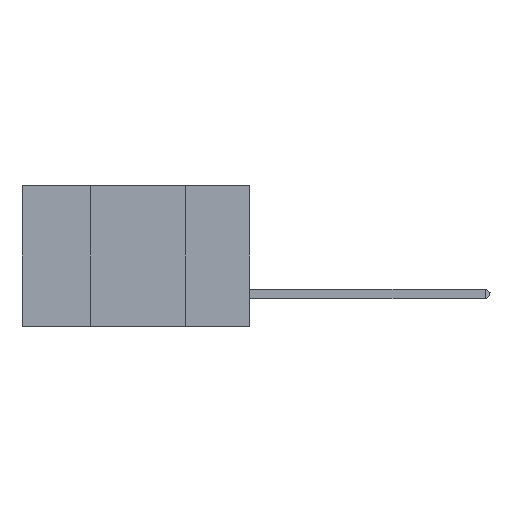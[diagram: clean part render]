
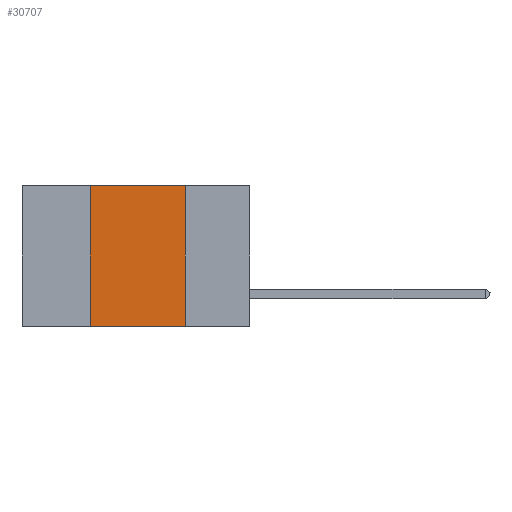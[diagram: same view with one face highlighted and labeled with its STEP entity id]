
A CAD part, left-side view. The second image highlights one B-rep face of the part: STEP entity #30707.
In plain terms, the highlighted planar face has unit normal (-1, 0, 0).
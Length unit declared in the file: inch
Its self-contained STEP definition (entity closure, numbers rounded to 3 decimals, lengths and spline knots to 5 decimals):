
#6168 = CARTESIAN_POINT ( 'NONE',  ( 0., 0.6, 0. ) ) ;
#6677 = ORIENTED_EDGE ( 'NONE', *, *, #27376, .F. ) ;
#6798 = VERTEX_POINT ( 'NONE', #9620 ) ;
#7410 = ORIENTED_EDGE ( 'NONE', *, *, #22093, .T. ) ;
#7739 = CARTESIAN_POINT ( 'NONE',  ( 0., 0.6, -0.37 ) ) ;
#8083 = CARTESIAN_POINT ( 'NONE',  ( 0., 0.17, 0. ) ) ;
#8646 = VERTEX_POINT ( 'NONE', #12746 ) ;
#9620 = CARTESIAN_POINT ( 'NONE',  ( 0., 0.42, 0. ) ) ;
#10170 = EDGE_CURVE ( 'NONE', #6798, #12693, #30324, .T. ) ;
#10676 = LINE ( 'NONE', #17947, #24309 ) ;
#11030 = VECTOR ( 'NONE', #15899, 39.37008 ) ;
#11172 = PLANE ( 'NONE',  #33672 ) ;
#12693 = VERTEX_POINT ( 'NONE', #8083 ) ;
#12746 = CARTESIAN_POINT ( 'NONE',  ( 0., 0.17, -0.37 ) ) ;
#14171 = DIRECTION ( 'NONE',  ( 0., 0., -1. ) ) ;
#14603 = VECTOR ( 'NONE', #25140, 39.37008 ) ;
#14664 = CARTESIAN_POINT ( 'NONE',  ( 0., 0.6, 0. ) ) ;
#15554 = ORIENTED_EDGE ( 'NONE', *, *, #22669, .F. ) ;
#15651 = EDGE_LOOP ( 'NONE', ( #15554, #31844, #6677, #7410 ) ) ;
#15899 = DIRECTION ( 'NONE',  ( 0., -1., 0. ) ) ;
#17947 = CARTESIAN_POINT ( 'NONE',  ( 0., 0.42, 0. ) ) ;
#18639 = FACE_OUTER_BOUND ( 'NONE', #15651, .T. ) ;
#20091 = LINE ( 'NONE', #23366, #29177 ) ;
#22093 = EDGE_CURVE ( 'NONE', #28716, #8646, #30490, .T. ) ;
#22669 = EDGE_CURVE ( 'NONE', #12693, #8646, #20091, .T. ) ;
#23366 = CARTESIAN_POINT ( 'NONE',  ( 0., 0.17, 0. ) ) ;
#24309 = VECTOR ( 'NONE', #33494, 39.37008 ) ;
#25140 = DIRECTION ( 'NONE',  ( 0., -1., 0. ) ) ;
#27085 = DIRECTION ( 'NONE',  ( 1., 0., 0. ) ) ;
#27376 = EDGE_CURVE ( 'NONE', #28716, #6798, #10676, .T. ) ;
#28623 = CARTESIAN_POINT ( 'NONE',  ( 0., 0.42, -0.37 ) ) ;
#28716 = VERTEX_POINT ( 'NONE', #28623 ) ;
#28737 = DIRECTION ( 'NONE',  ( 0., 0., -1. ) ) ;
#29177 = VECTOR ( 'NONE', #28737, 39.37008 ) ;
#30324 = LINE ( 'NONE', #14664, #14603 ) ;
#30490 = LINE ( 'NONE', #7739, #11030 ) ;
#30707 = ADVANCED_FACE ( 'NONE', ( #18639 ), #11172, .F. ) ;
#31844 = ORIENTED_EDGE ( 'NONE', *, *, #10170, .F. ) ;
#33494 = DIRECTION ( 'NONE',  ( 0., 0., 1. ) ) ;
#33672 = AXIS2_PLACEMENT_3D ( 'NONE', #6168, #27085, #14171 ) ;
